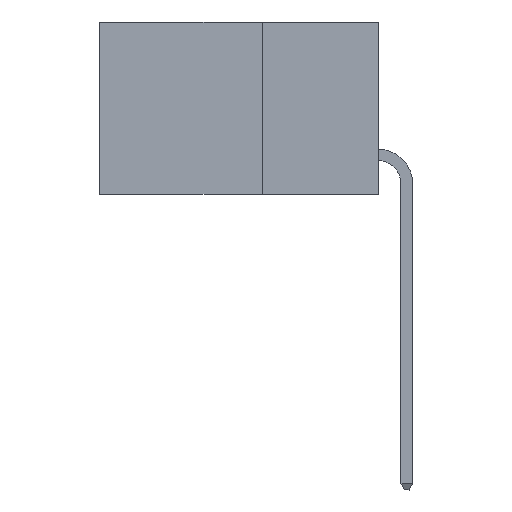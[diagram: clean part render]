
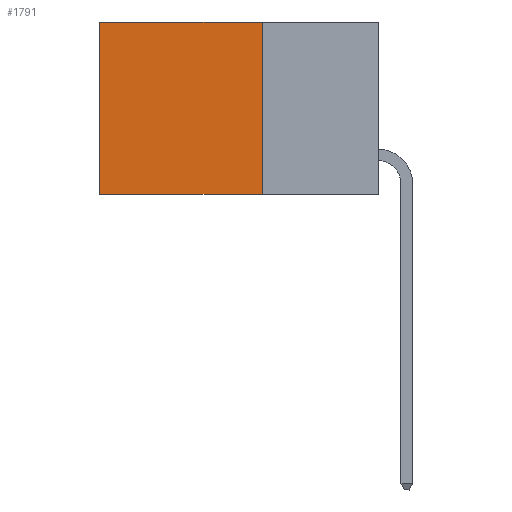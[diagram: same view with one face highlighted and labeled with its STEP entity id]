
A CAD part, left-side view. The second image highlights one B-rep face of the part: STEP entity #1791.
In plain terms, the highlighted planar face has unit normal (-1, 0, 0).
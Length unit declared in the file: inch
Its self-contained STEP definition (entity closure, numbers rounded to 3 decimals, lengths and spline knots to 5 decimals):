
#36 = CARTESIAN_POINT ( 'NONE',  ( 0.2615, 0.6, 0. ) ) ;
#590 = CARTESIAN_POINT ( 'NONE',  ( 0.2615, 0.25, -0.37 ) ) ;
#925 = CARTESIAN_POINT ( 'NONE',  ( 0.2615, 0.25, 0. ) ) ;
#1437 = DIRECTION ( 'NONE',  ( 1., 0., 0. ) ) ;
#1791 = ADVANCED_FACE ( 'NONE', ( #6632 ), #5496, .F. ) ;
#2026 = CARTESIAN_POINT ( 'NONE',  ( 0.2615, 0.6, -0.37 ) ) ;
#2411 = EDGE_CURVE ( 'NONE', #3279, #4432, #7777, .T. ) ;
#2658 = VERTEX_POINT ( 'NONE', #11294 ) ;
#2863 = LINE ( 'NONE', #2026, #10911 ) ;
#3279 = VERTEX_POINT ( 'NONE', #8859 ) ;
#3503 = LINE ( 'NONE', #10215, #7548 ) ;
#3582 = DIRECTION ( 'NONE',  ( 0., 0., -1. ) ) ;
#3736 = ORIENTED_EDGE ( 'NONE', *, *, #11884, .T. ) ;
#3955 = ORIENTED_EDGE ( 'NONE', *, *, #2411, .F. ) ;
#4022 = ORIENTED_EDGE ( 'NONE', *, *, #9389, .F. ) ;
#4432 = VERTEX_POINT ( 'NONE', #8359 ) ;
#4768 = ORIENTED_EDGE ( 'NONE', *, *, #11850, .T. ) ;
#4863 = LINE ( 'NONE', #925, #5129 ) ;
#5129 = VECTOR ( 'NONE', #8797, 39.37008 ) ;
#5496 = PLANE ( 'NONE',  #6865 ) ;
#5727 = CARTESIAN_POINT ( 'NONE',  ( 0.2615, 0.25, -0.37 ) ) ;
#5782 = VERTEX_POINT ( 'NONE', #36 ) ;
#6445 = DIRECTION ( 'NONE',  ( 0., 0., -1. ) ) ;
#6632 = FACE_OUTER_BOUND ( 'NONE', #8333, .T. ) ;
#6865 = AXIS2_PLACEMENT_3D ( 'NONE', #590, #1437, #3582 ) ;
#7548 = VECTOR ( 'NONE', #6445, 39.37008 ) ;
#7777 = LINE ( 'NONE', #5727, #8611 ) ;
#8333 = EDGE_LOOP ( 'NONE', ( #3736, #3955, #4022, #4768 ) ) ;
#8359 = CARTESIAN_POINT ( 'NONE',  ( 0.2615, 0.6, -0.37 ) ) ;
#8611 = VECTOR ( 'NONE', #12593, 39.37008 ) ;
#8797 = DIRECTION ( 'NONE',  ( 0., 1., 0. ) ) ;
#8859 = CARTESIAN_POINT ( 'NONE',  ( 0.2615, 0.25, -0.37 ) ) ;
#9389 = EDGE_CURVE ( 'NONE', #2658, #3279, #3503, .T. ) ;
#10215 = CARTESIAN_POINT ( 'NONE',  ( 0.2615, 0.25, -0.37 ) ) ;
#10911 = VECTOR ( 'NONE', #11653, 39.37008 ) ;
#11294 = CARTESIAN_POINT ( 'NONE',  ( 0.2615, 0.25, 0. ) ) ;
#11653 = DIRECTION ( 'NONE',  ( 0., 0., -1. ) ) ;
#11850 = EDGE_CURVE ( 'NONE', #2658, #5782, #4863, .T. ) ;
#11884 = EDGE_CURVE ( 'NONE', #5782, #4432, #2863, .T. ) ;
#12593 = DIRECTION ( 'NONE',  ( 0., 1., 0. ) ) ;
